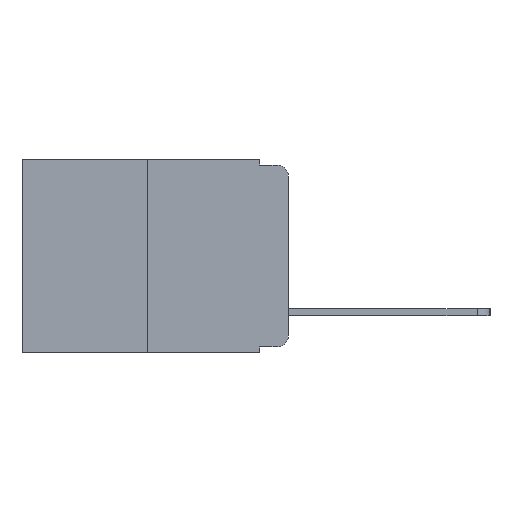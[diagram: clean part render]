
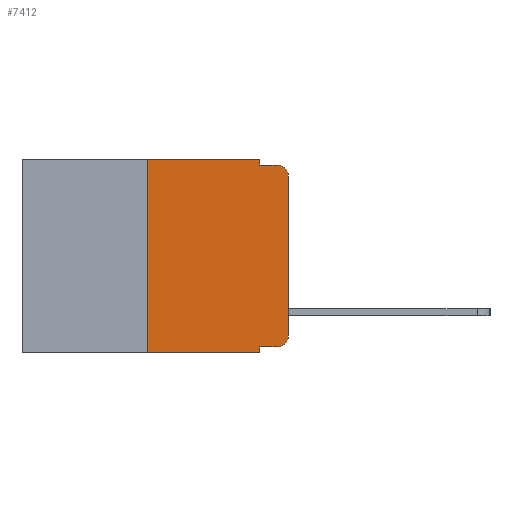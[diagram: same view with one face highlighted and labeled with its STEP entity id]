
A CAD part, left-side view. The second image highlights one B-rep face of the part: STEP entity #7412.
In plain terms, the highlighted planar face has unit normal (-1, 0, 0).
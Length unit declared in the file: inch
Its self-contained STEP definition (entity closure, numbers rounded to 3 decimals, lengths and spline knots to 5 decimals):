
#279 = VECTOR ( 'NONE', #4118, 39.37008 ) ;
#482 = DIRECTION ( 'NONE',  ( 0., 0., 1. ) ) ;
#489 = VECTOR ( 'NONE', #482, 39.37008 ) ;
#772 = DIRECTION ( 'NONE',  ( 0., 0., -1. ) ) ;
#1069 = ORIENTED_EDGE ( 'NONE', *, *, #12204, .T. ) ;
#1208 = CARTESIAN_POINT ( 'NONE',  ( 0., 0.051, 0. ) ) ;
#1283 = EDGE_CURVE ( 'NONE', #1598, #2016, #14285, .T. ) ;
#1557 = DIRECTION ( 'NONE',  ( 0., -1., 0. ) ) ;
#1598 = VERTEX_POINT ( 'NONE', #13663 ) ;
#2016 = VERTEX_POINT ( 'NONE', #11107 ) ;
#2111 = LINE ( 'NONE', #9496, #11804 ) ;
#2382 = DIRECTION ( 'NONE',  ( -1., 0., 0. ) ) ;
#2699 = DIRECTION ( 'NONE',  ( 0., -1., 0. ) ) ;
#2763 = EDGE_CURVE ( 'NONE', #14895, #12446, #13554, .T. ) ;
#3303 = CARTESIAN_POINT ( 'NONE',  ( 0., 0.02, -0.01 ) ) ;
#3316 = DIRECTION ( 'NONE',  ( 1., 0., 0. ) ) ;
#4118 = DIRECTION ( 'NONE',  ( 0., -1., 0. ) ) ;
#4385 = ORIENTED_EDGE ( 'NONE', *, *, #6285, .F. ) ;
#4734 = VERTEX_POINT ( 'NONE', #3303 ) ;
#4781 = VERTEX_POINT ( 'NONE', #15613 ) ;
#4868 = EDGE_CURVE ( 'NONE', #11425, #4781, #9912, .T. ) ;
#4954 = LINE ( 'NONE', #11488, #7637 ) ;
#4958 = EDGE_CURVE ( 'NONE', #4781, #4734, #5787, .T. ) ;
#5383 = ORIENTED_EDGE ( 'NONE', *, *, #4958, .T. ) ;
#5787 = CIRCLE ( 'NONE', #12846, 0.02 ) ;
#5821 = CARTESIAN_POINT ( 'NONE',  ( 0., 0.051, -0.333 ) ) ;
#5860 = CARTESIAN_POINT ( 'NONE',  ( 0., 0.051, -0.01 ) ) ;
#5862 = PLANE ( 'NONE',  #9495 ) ;
#5893 = CARTESIAN_POINT ( 'NONE',  ( 0., 0.02, -0.333 ) ) ;
#6241 = VERTEX_POINT ( 'NONE', #5860 ) ;
#6285 = EDGE_CURVE ( 'NONE', #15087, #1598, #7827, .T. ) ;
#6325 = CARTESIAN_POINT ( 'NONE',  ( 0., 0.051, 0. ) ) ;
#6344 = VECTOR ( 'NONE', #11518, 39.37008 ) ;
#6627 = VECTOR ( 'NONE', #12222, 39.37008 ) ;
#7412 = ADVANCED_FACE ( 'NONE', ( #12436 ), #5862, .F. ) ;
#7505 = LINE ( 'NONE', #15285, #13464 ) ;
#7599 = DIRECTION ( 'NONE',  ( -1., 0., 0. ) ) ;
#7637 = VECTOR ( 'NONE', #2699, 39.37008 ) ;
#7827 = LINE ( 'NONE', #15683, #489 ) ;
#8260 = ORIENTED_EDGE ( 'NONE', *, *, #2763, .F. ) ;
#9067 = EDGE_CURVE ( 'NONE', #6241, #4734, #2111, .T. ) ;
#9495 = AXIS2_PLACEMENT_3D ( 'NONE', #10829, #3316, #12023 ) ;
#9496 = CARTESIAN_POINT ( 'NONE',  ( 0., 0.051, -0.01 ) ) ;
#9533 = ORIENTED_EDGE ( 'NONE', *, *, #9067, .F. ) ;
#9912 = LINE ( 'NONE', #11034, #6627 ) ;
#10048 = CARTESIAN_POINT ( 'NONE',  ( 0., 0.02, -0.313 ) ) ;
#10394 = CARTESIAN_POINT ( 'NONE',  ( 0., 0., -0.313 ) ) ;
#10455 = VECTOR ( 'NONE', #772, 39.37008 ) ;
#10670 = DIRECTION ( 'NONE',  ( 0., -1., 0. ) ) ;
#10806 = ORIENTED_EDGE ( 'NONE', *, *, #4868, .T. ) ;
#10826 = LINE ( 'NONE', #6325, #10455 ) ;
#10829 = CARTESIAN_POINT ( 'NONE',  ( 0., 0.473, 0. ) ) ;
#10840 = EDGE_LOOP ( 'NONE', ( #10806, #5383, #9533, #13430, #13778, #4385, #1069, #8260, #12122, #12889 ) ) ;
#11034 = CARTESIAN_POINT ( 'NONE',  ( 0., 0., 0. ) ) ;
#11107 = CARTESIAN_POINT ( 'NONE',  ( 0., 0.051, 0. ) ) ;
#11223 = DIRECTION ( 'NONE',  ( 0., 0., -1. ) ) ;
#11425 = VERTEX_POINT ( 'NONE', #10394 ) ;
#11488 = CARTESIAN_POINT ( 'NONE',  ( 0., 0.051, -0.333 ) ) ;
#11518 = DIRECTION ( 'NONE',  ( 0., 0., -1. ) ) ;
#11560 = VERTEX_POINT ( 'NONE', #5893 ) ;
#11804 = VECTOR ( 'NONE', #10670, 39.37008 ) ;
#12023 = DIRECTION ( 'NONE',  ( 0., 0., -1. ) ) ;
#12122 = ORIENTED_EDGE ( 'NONE', *, *, #15806, .T. ) ;
#12204 = EDGE_CURVE ( 'NONE', #15087, #12446, #7505, .T. ) ;
#12222 = DIRECTION ( 'NONE',  ( 0., 0., 1. ) ) ;
#12436 = FACE_OUTER_BOUND ( 'NONE', #10840, .T. ) ;
#12446 = VERTEX_POINT ( 'NONE', #14607 ) ;
#12816 = EDGE_CURVE ( 'NONE', #2016, #6241, #10826, .T. ) ;
#12846 = AXIS2_PLACEMENT_3D ( 'NONE', #14678, #7599, #15875 ) ;
#12889 = ORIENTED_EDGE ( 'NONE', *, *, #14510, .T. ) ;
#13430 = ORIENTED_EDGE ( 'NONE', *, *, #12816, .F. ) ;
#13464 = VECTOR ( 'NONE', #1557, 39.37008 ) ;
#13554 = LINE ( 'NONE', #1208, #6344 ) ;
#13663 = CARTESIAN_POINT ( 'NONE',  ( 0., 0.25, 0. ) ) ;
#13778 = ORIENTED_EDGE ( 'NONE', *, *, #1283, .F. ) ;
#14066 = AXIS2_PLACEMENT_3D ( 'NONE', #10048, #2382, #11223 ) ;
#14285 = LINE ( 'NONE', #16233, #279 ) ;
#14510 = EDGE_CURVE ( 'NONE', #11560, #11425, #14704, .T. ) ;
#14607 = CARTESIAN_POINT ( 'NONE',  ( 0., 0.051, -0.343 ) ) ;
#14678 = CARTESIAN_POINT ( 'NONE',  ( 0., 0.02, -0.03 ) ) ;
#14704 = CIRCLE ( 'NONE', #14066, 0.02 ) ;
#14895 = VERTEX_POINT ( 'NONE', #5821 ) ;
#15087 = VERTEX_POINT ( 'NONE', #15847 ) ;
#15285 = CARTESIAN_POINT ( 'NONE',  ( 0., 0.473, -0.343 ) ) ;
#15613 = CARTESIAN_POINT ( 'NONE',  ( 0., 0., -0.03 ) ) ;
#15683 = CARTESIAN_POINT ( 'NONE',  ( 0., 0.25, 0. ) ) ;
#15806 = EDGE_CURVE ( 'NONE', #14895, #11560, #4954, .T. ) ;
#15847 = CARTESIAN_POINT ( 'NONE',  ( 0., 0.25, -0.343 ) ) ;
#15875 = DIRECTION ( 'NONE',  ( 0., 0., -1. ) ) ;
#16233 = CARTESIAN_POINT ( 'NONE',  ( 0., 0.473, 0. ) ) ;
